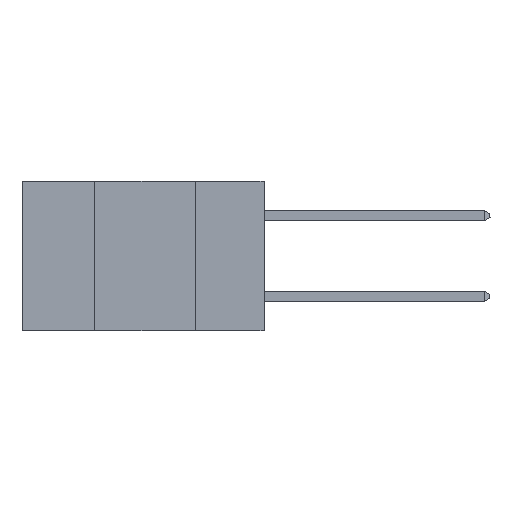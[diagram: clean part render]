
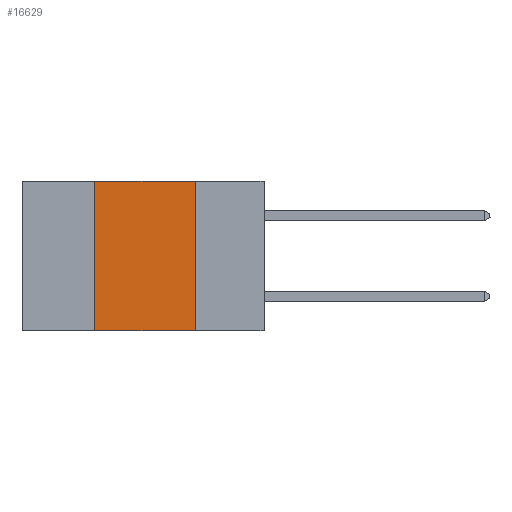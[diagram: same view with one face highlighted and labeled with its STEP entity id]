
A CAD part, left-side view. The second image highlights one B-rep face of the part: STEP entity #16629.
In plain terms, the highlighted planar face has unit normal (-1, 0, 0).
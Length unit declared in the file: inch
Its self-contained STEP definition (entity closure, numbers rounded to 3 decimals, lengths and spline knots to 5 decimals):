
#229 = DIRECTION ( 'NONE',  ( 1., 0., 0. ) ) ;
#730 = DIRECTION ( 'NONE',  ( 0., -1., 0. ) ) ;
#933 = CARTESIAN_POINT ( 'NONE',  ( 0., 0.17, 0. ) ) ;
#1485 = ORIENTED_EDGE ( 'NONE', *, *, #3626, .F. ) ;
#1682 = VERTEX_POINT ( 'NONE', #14756 ) ;
#2521 = CARTESIAN_POINT ( 'NONE',  ( 0., 0.17, 0. ) ) ;
#2743 = DIRECTION ( 'NONE',  ( 0., -1., 0. ) ) ;
#3125 = EDGE_CURVE ( 'NONE', #16844, #1682, #4723, .T. ) ;
#3411 = EDGE_CURVE ( 'NONE', #16436, #1682, #12814, .T. ) ;
#3626 = EDGE_CURVE ( 'NONE', #13409, #16844, #10117, .T. ) ;
#4510 = VECTOR ( 'NONE', #2743, 39.37008 ) ;
#4575 = ORIENTED_EDGE ( 'NONE', *, *, #11016, .F. ) ;
#4723 = LINE ( 'NONE', #2521, #9516 ) ;
#4772 = EDGE_LOOP ( 'NONE', ( #11032, #1485, #4575, #8969 ) ) ;
#5569 = PLANE ( 'NONE',  #17103 ) ;
#6777 = CARTESIAN_POINT ( 'NONE',  ( 0., 0.6, -0.37 ) ) ;
#6925 = CARTESIAN_POINT ( 'NONE',  ( 0., 0.6, 0. ) ) ;
#7142 = FACE_OUTER_BOUND ( 'NONE', #4772, .T. ) ;
#8463 = LINE ( 'NONE', #17091, #13208 ) ;
#8969 = ORIENTED_EDGE ( 'NONE', *, *, #3411, .T. ) ;
#9288 = CARTESIAN_POINT ( 'NONE',  ( 0., 0.42, -0.37 ) ) ;
#9516 = VECTOR ( 'NONE', #10249, 39.37008 ) ;
#10117 = LINE ( 'NONE', #11376, #12400 ) ;
#10249 = DIRECTION ( 'NONE',  ( 0., 0., -1. ) ) ;
#11016 = EDGE_CURVE ( 'NONE', #16436, #13409, #8463, .T. ) ;
#11032 = ORIENTED_EDGE ( 'NONE', *, *, #3125, .F. ) ;
#11376 = CARTESIAN_POINT ( 'NONE',  ( 0., 0.6, 0. ) ) ;
#12400 = VECTOR ( 'NONE', #730, 39.37008 ) ;
#12814 = LINE ( 'NONE', #6777, #4510 ) ;
#12880 = DIRECTION ( 'NONE',  ( 0., 0., 1. ) ) ;
#13208 = VECTOR ( 'NONE', #12880, 39.37008 ) ;
#13409 = VERTEX_POINT ( 'NONE', #13460 ) ;
#13460 = CARTESIAN_POINT ( 'NONE',  ( 0., 0.42, 0. ) ) ;
#14756 = CARTESIAN_POINT ( 'NONE',  ( 0., 0.17, -0.37 ) ) ;
#14896 = DIRECTION ( 'NONE',  ( 0., 0., -1. ) ) ;
#16436 = VERTEX_POINT ( 'NONE', #9288 ) ;
#16629 = ADVANCED_FACE ( 'NONE', ( #7142 ), #5569, .F. ) ;
#16844 = VERTEX_POINT ( 'NONE', #933 ) ;
#17091 = CARTESIAN_POINT ( 'NONE',  ( 0., 0.42, 0. ) ) ;
#17103 = AXIS2_PLACEMENT_3D ( 'NONE', #6925, #229, #14896 ) ;
